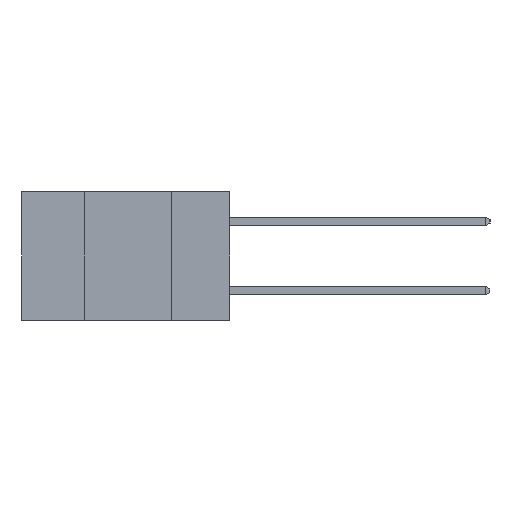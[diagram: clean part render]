
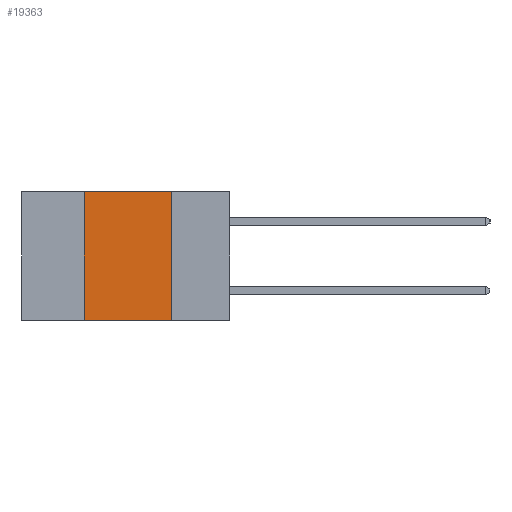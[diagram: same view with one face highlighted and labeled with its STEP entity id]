
A CAD part, left-side view. The second image highlights one B-rep face of the part: STEP entity #19363.
In plain terms, the highlighted planar face has unit normal (-1, 0, 0).
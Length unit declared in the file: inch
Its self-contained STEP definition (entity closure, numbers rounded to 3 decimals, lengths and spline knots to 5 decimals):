
#7 = CARTESIAN_POINT ( 'NONE',  ( 0., 0.42, 0. ) ) ;
#357 = CARTESIAN_POINT ( 'NONE',  ( 0., 0.6, 0. ) ) ;
#709 = ORIENTED_EDGE ( 'NONE', *, *, #6637, .F. ) ;
#1242 = DIRECTION ( 'NONE',  ( 0., 0., 1. ) ) ;
#1309 = DIRECTION ( 'NONE',  ( 0., 0., -1. ) ) ;
#1320 = CARTESIAN_POINT ( 'NONE',  ( 0., 0.42, -0.37 ) ) ;
#2147 = DIRECTION ( 'NONE',  ( 0., -1., 0. ) ) ;
#2514 = VECTOR ( 'NONE', #1242, 39.37008 ) ;
#3765 = ORIENTED_EDGE ( 'NONE', *, *, #12608, .F. ) ;
#4319 = ORIENTED_EDGE ( 'NONE', *, *, #13778, .F. ) ;
#4453 = CARTESIAN_POINT ( 'NONE',  ( 0., 0.17, 0. ) ) ;
#4560 = LINE ( 'NONE', #6538, #17934 ) ;
#4878 = LINE ( 'NONE', #357, #18797 ) ;
#6538 = CARTESIAN_POINT ( 'NONE',  ( 0., 0.17, -0.37 ) ) ;
#6637 = EDGE_CURVE ( 'NONE', #11473, #9245, #21048, .T. ) ;
#7680 = CARTESIAN_POINT ( 'NONE',  ( 0., 0.6, -0.37 ) ) ;
#9245 = VERTEX_POINT ( 'NONE', #7 ) ;
#9552 = DIRECTION ( 'NONE',  ( 0., 0., -1. ) ) ;
#10418 = EDGE_LOOP ( 'NONE', ( #4319, #3765, #709, #18224 ) ) ;
#11342 = VERTEX_POINT ( 'NONE', #4453 ) ;
#11473 = VERTEX_POINT ( 'NONE', #13469 ) ;
#12060 = EDGE_CURVE ( 'NONE', #11473, #13724, #20407, .T. ) ;
#12608 = EDGE_CURVE ( 'NONE', #9245, #11342, #4878, .T. ) ;
#12645 = AXIS2_PLACEMENT_3D ( 'NONE', #18235, #19973, #9552 ) ;
#13469 = CARTESIAN_POINT ( 'NONE',  ( 0., 0.42, -0.37 ) ) ;
#13724 = VERTEX_POINT ( 'NONE', #16916 ) ;
#13778 = EDGE_CURVE ( 'NONE', #11342, #13724, #4560, .T. ) ;
#14721 = DIRECTION ( 'NONE',  ( 0., -1., 0. ) ) ;
#15835 = VECTOR ( 'NONE', #14721, 39.37008 ) ;
#16491 = PLANE ( 'NONE',  #12645 ) ;
#16916 = CARTESIAN_POINT ( 'NONE',  ( 0., 0.17, -0.37 ) ) ;
#17934 = VECTOR ( 'NONE', #1309, 39.37008 ) ;
#18224 = ORIENTED_EDGE ( 'NONE', *, *, #12060, .T. ) ;
#18235 = CARTESIAN_POINT ( 'NONE',  ( 0., 0.6, 0. ) ) ;
#18797 = VECTOR ( 'NONE', #2147, 39.37008 ) ;
#19363 = ADVANCED_FACE ( 'NONE', ( #21997 ), #16491, .F. ) ;
#19973 = DIRECTION ( 'NONE',  ( 1., 0., 0. ) ) ;
#20407 = LINE ( 'NONE', #7680, #15835 ) ;
#21048 = LINE ( 'NONE', #1320, #2514 ) ;
#21997 = FACE_OUTER_BOUND ( 'NONE', #10418, .T. ) ;
